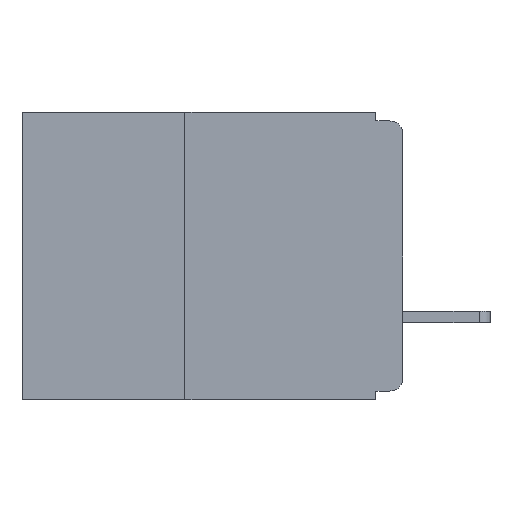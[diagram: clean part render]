
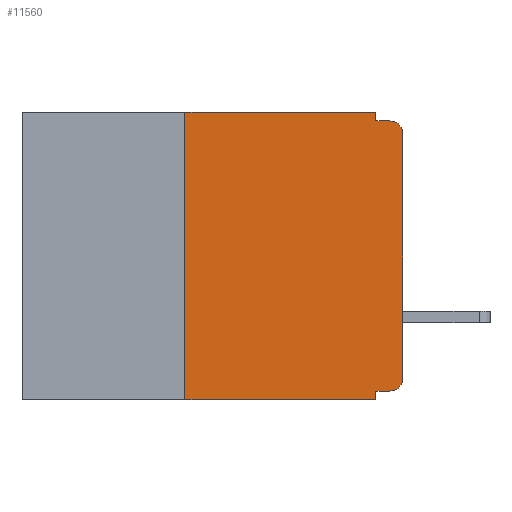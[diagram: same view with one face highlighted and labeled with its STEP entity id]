
A CAD part, left-side view. The second image highlights one B-rep face of the part: STEP entity #11560.
In plain terms, the highlighted planar face has unit normal (-1, 0, 0).
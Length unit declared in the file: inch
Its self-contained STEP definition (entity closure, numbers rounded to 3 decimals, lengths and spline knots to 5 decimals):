
#285 = DIRECTION ( 'NONE',  ( 0., -1., 0. ) ) ;
#697 = AXIS2_PLACEMENT_3D ( 'NONE', #9341, #9205, #9174 ) ;
#768 = VERTEX_POINT ( 'NONE', #26592 ) ;
#2289 = LINE ( 'NONE', #31570, #17461 ) ;
#2781 = PLANE ( 'NONE',  #32680 ) ;
#2872 = CARTESIAN_POINT ( 'NONE',  ( 0., 0.031, -0.33 ) ) ;
#3417 = CARTESIAN_POINT ( 'NONE',  ( 0., 0.031, -0.01 ) ) ;
#4053 = ORIENTED_EDGE ( 'NONE', *, *, #6856, .F. ) ;
#4990 = EDGE_LOOP ( 'NONE', ( #31786, #24228, #4053, #15832, #33090, #16657, #9829, #28068, #21419, #18943 ) ) ;
#5012 = EDGE_CURVE ( 'NONE', #22094, #23800, #25736, .T. ) ;
#5056 = CARTESIAN_POINT ( 'NONE',  ( 0., 0., 0. ) ) ;
#5560 = DIRECTION ( 'NONE',  ( 1., 0., 0. ) ) ;
#5565 = LINE ( 'NONE', #7021, #32667 ) ;
#6787 = DIRECTION ( 'NONE',  ( 0., -1., 0. ) ) ;
#6816 = EDGE_CURVE ( 'NONE', #22094, #18729, #8124, .T. ) ;
#6856 = EDGE_CURVE ( 'NONE', #23838, #18766, #5565, .T. ) ;
#7021 = CARTESIAN_POINT ( 'NONE',  ( 0., 0., -0.01 ) ) ;
#8000 = CARTESIAN_POINT ( 'NONE',  ( 0., 0., -0.305 ) ) ;
#8059 = CARTESIAN_POINT ( 'NONE',  ( 0., 0.031, 0. ) ) ;
#8124 = CIRCLE ( 'NONE', #697, 0.015 ) ;
#8495 = DIRECTION ( 'NONE',  ( 0., 0., 1. ) ) ;
#9174 = DIRECTION ( 'NONE',  ( 0., 0., -1. ) ) ;
#9205 = DIRECTION ( 'NONE',  ( -1., 0., 0. ) ) ;
#9256 = VECTOR ( 'NONE', #31835, 39.37008 ) ;
#9341 = CARTESIAN_POINT ( 'NONE',  ( 0., 0.015, -0.305 ) ) ;
#9829 = ORIENTED_EDGE ( 'NONE', *, *, #13262, .T. ) ;
#10348 = EDGE_CURVE ( 'NONE', #18729, #17240, #30898, .T. ) ;
#11528 = CARTESIAN_POINT ( 'NONE',  ( 0., 0.015, -0.01 ) ) ;
#11560 = ADVANCED_FACE ( 'NONE', ( #19442 ), #2781, .F. ) ;
#12700 = EDGE_CURVE ( 'NONE', #22295, #14861, #21593, .T. ) ;
#12798 = CIRCLE ( 'NONE', #29206, 0.015 ) ;
#12929 = VECTOR ( 'NONE', #21566, 39.37008 ) ;
#13262 = EDGE_CURVE ( 'NONE', #22295, #768, #2289, .T. ) ;
#13456 = VECTOR ( 'NONE', #21948, 39.37008 ) ;
#13796 = VECTOR ( 'NONE', #8495, 39.37008 ) ;
#13927 = VERTEX_POINT ( 'NONE', #8059 ) ;
#14066 = CARTESIAN_POINT ( 'NONE',  ( 0., 0.031, -0.32 ) ) ;
#14116 = CARTESIAN_POINT ( 'NONE',  ( 0., 0.015, -0.025 ) ) ;
#14340 = LINE ( 'NONE', #19082, #27387 ) ;
#14861 = VERTEX_POINT ( 'NONE', #20650 ) ;
#15832 = ORIENTED_EDGE ( 'NONE', *, *, #25590, .F. ) ;
#16657 = ORIENTED_EDGE ( 'NONE', *, *, #12700, .F. ) ;
#16741 = DIRECTION ( 'NONE',  ( 0., 0., -1. ) ) ;
#17240 = VERTEX_POINT ( 'NONE', #22141 ) ;
#17461 = VECTOR ( 'NONE', #18658, 39.37008 ) ;
#18351 = DIRECTION ( 'NONE',  ( 0., 0., 1. ) ) ;
#18658 = DIRECTION ( 'NONE',  ( 0., -1., 0. ) ) ;
#18729 = VERTEX_POINT ( 'NONE', #8000 ) ;
#18737 = EDGE_CURVE ( 'NONE', #17240, #18766, #12798, .T. ) ;
#18766 = VERTEX_POINT ( 'NONE', #11528 ) ;
#18821 = CARTESIAN_POINT ( 'NONE',  ( 0., 0.031, 0. ) ) ;
#18851 = CARTESIAN_POINT ( 'NONE',  ( 0., 0.437, 0. ) ) ;
#18943 = ORIENTED_EDGE ( 'NONE', *, *, #6816, .T. ) ;
#19082 = CARTESIAN_POINT ( 'NONE',  ( 0., 0.437, 0. ) ) ;
#19442 = FACE_OUTER_BOUND ( 'NONE', #4990, .T. ) ;
#20650 = CARTESIAN_POINT ( 'NONE',  ( 0., 0.25, 0. ) ) ;
#21419 = ORIENTED_EDGE ( 'NONE', *, *, #5012, .F. ) ;
#21566 = DIRECTION ( 'NONE',  ( 0., 0., -1. ) ) ;
#21593 = LINE ( 'NONE', #26915, #13796 ) ;
#21622 = CARTESIAN_POINT ( 'NONE',  ( 0., 0., -0.32 ) ) ;
#21948 = DIRECTION ( 'NONE',  ( 0., 1., 0. ) ) ;
#22094 = VERTEX_POINT ( 'NONE', #24781 ) ;
#22141 = CARTESIAN_POINT ( 'NONE',  ( 0., 0., -0.025 ) ) ;
#22295 = VERTEX_POINT ( 'NONE', #23083 ) ;
#23083 = CARTESIAN_POINT ( 'NONE',  ( 0., 0.25, -0.33 ) ) ;
#23302 = LINE ( 'NONE', #18821, #9256 ) ;
#23800 = VERTEX_POINT ( 'NONE', #14066 ) ;
#23838 = VERTEX_POINT ( 'NONE', #3417 ) ;
#24098 = DIRECTION ( 'NONE',  ( 0., 0., -1. ) ) ;
#24228 = ORIENTED_EDGE ( 'NONE', *, *, #18737, .T. ) ;
#24781 = CARTESIAN_POINT ( 'NONE',  ( 0., 0.015, -0.32 ) ) ;
#25010 = EDGE_CURVE ( 'NONE', #14861, #13927, #14340, .T. ) ;
#25590 = EDGE_CURVE ( 'NONE', #13927, #23838, #23302, .T. ) ;
#25736 = LINE ( 'NONE', #21622, #13456 ) ;
#26592 = CARTESIAN_POINT ( 'NONE',  ( 0., 0.031, -0.33 ) ) ;
#26857 = LINE ( 'NONE', #2872, #12929 ) ;
#26915 = CARTESIAN_POINT ( 'NONE',  ( 0., 0.25, -0.33 ) ) ;
#27387 = VECTOR ( 'NONE', #285, 39.37008 ) ;
#28068 = ORIENTED_EDGE ( 'NONE', *, *, #34183, .F. ) ;
#29206 = AXIS2_PLACEMENT_3D ( 'NONE', #14116, #32261, #16741 ) ;
#30098 = VECTOR ( 'NONE', #18351, 39.37008 ) ;
#30898 = LINE ( 'NONE', #5056, #30098 ) ;
#31570 = CARTESIAN_POINT ( 'NONE',  ( 0., 0.437, -0.33 ) ) ;
#31786 = ORIENTED_EDGE ( 'NONE', *, *, #10348, .T. ) ;
#31835 = DIRECTION ( 'NONE',  ( 0., 0., -1. ) ) ;
#32261 = DIRECTION ( 'NONE',  ( -1., 0., 0. ) ) ;
#32667 = VECTOR ( 'NONE', #6787, 39.37008 ) ;
#32680 = AXIS2_PLACEMENT_3D ( 'NONE', #18851, #5560, #24098 ) ;
#33090 = ORIENTED_EDGE ( 'NONE', *, *, #25010, .F. ) ;
#34183 = EDGE_CURVE ( 'NONE', #23800, #768, #26857, .T. ) ;
